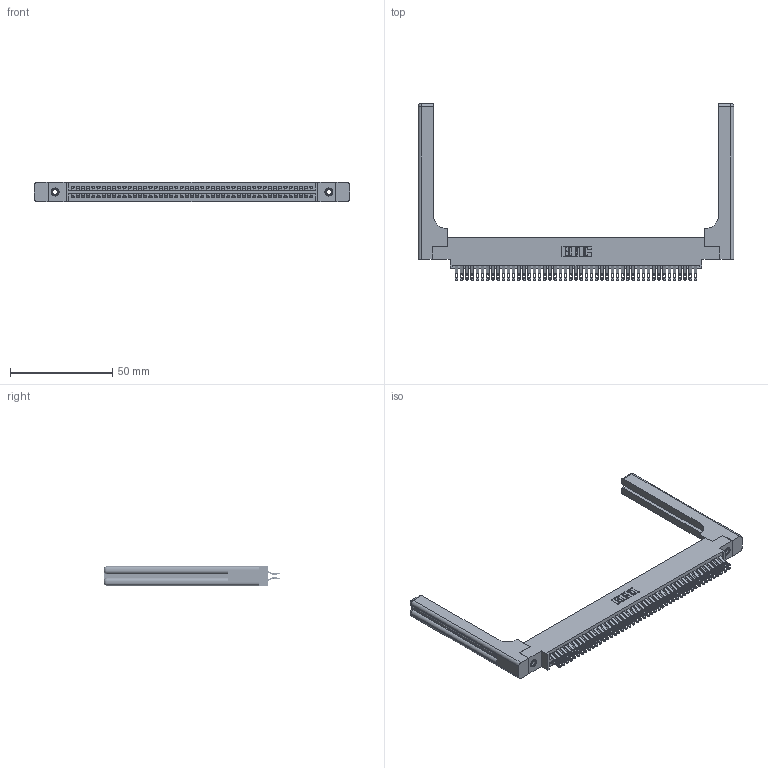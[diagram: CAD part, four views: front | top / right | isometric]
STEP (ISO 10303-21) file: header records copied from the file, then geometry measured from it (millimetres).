
FILE_DESCRIPTION (( 'STEP AP203' ), '1' );
FILE_NAME ('345-094-555-858.STEP', '2019-11-02T05:31:43', ( '' ), ( '' ), 'SwSTEP 2.0', 'SolidWorks 2016', '' );
FILE_SCHEMA (( 'CONFIG_CONTROL_DESIGN' ));
Length unit declared in the file: inch
Products named in the file (5): 345-292-001_555 Tail; 345-094-555-858; 345 Part_0.170 Offset - 0.156 Dia-TH; 345-220-058_345-220-058; 345-250-001_345-250-001-102
Assembly tree (99 placements, depth 2):
  345-094-555-858
    345 Part_0.170 Offset - 0.156 Dia-TH
    345-292-001_555 Tail  x94
    345-250-001_345-250-001-102  x2
    345-220-058_345-220-058  x2
Bounding box: 154.41 x 86.41 x 9.4 mm (x, y, z)
Volume: 23680 mm3; surface area: 28722.9 mm2
Topology: 99 solids, 99 shells, 5650 faces, 17657 edges, 11750 vertices
Faces by surface type: plane 3146, cylinder 2444, bspline 36, cone 12, sphere 8, torus 4
Entity records: 41844 total; most frequent: CARTESIAN_POINT 8039, ORIENTED_EDGE 6740, DIRECTION 5982, EDGE_CURVE 3370, VECTOR 2938, LINE 2938, VERTEX_POINT 2238, AXIS2_PLACEMENT_3D 1522
